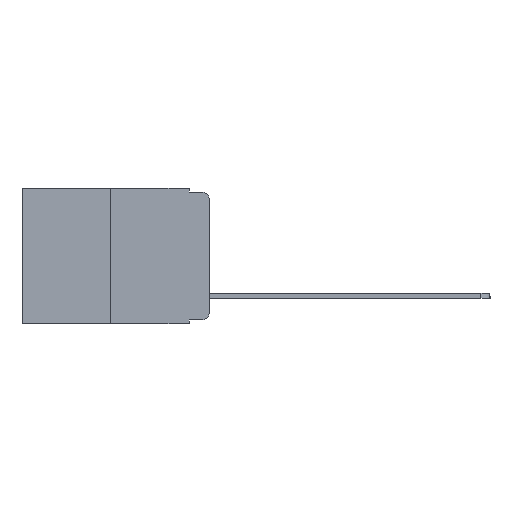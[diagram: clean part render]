
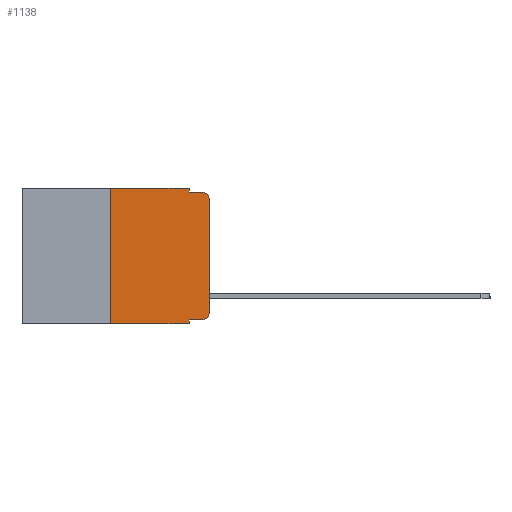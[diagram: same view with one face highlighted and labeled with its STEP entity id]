
A CAD part, left-side view. The second image highlights one B-rep face of the part: STEP entity #1138.
In plain terms, the highlighted planar face has unit normal (-1, 0, 0).
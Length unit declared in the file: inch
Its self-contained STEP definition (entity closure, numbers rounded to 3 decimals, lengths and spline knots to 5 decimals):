
#285 = VECTOR ( 'NONE', #13796, 39.37008 ) ;
#862 = ORIENTED_EDGE ( 'NONE', *, *, #1013, .T. ) ;
#1013 = EDGE_CURVE ( 'NONE', #11728, #10375, #12102, .T. ) ;
#1138 = ADVANCED_FACE ( 'NONE', ( #19565 ), #14277, .F. ) ;
#1579 = DIRECTION ( 'NONE',  ( -1., 0., 0. ) ) ;
#1779 = ORIENTED_EDGE ( 'NONE', *, *, #4696, .T. ) ;
#1938 = CARTESIAN_POINT ( 'NONE',  ( 0., 0.02, -0.333 ) ) ;
#2696 = EDGE_CURVE ( 'NONE', #3212, #5462, #18190, .T. ) ;
#2874 = CARTESIAN_POINT ( 'NONE',  ( 0., 0.051, -0.333 ) ) ;
#3212 = VERTEX_POINT ( 'NONE', #9689 ) ;
#3411 = DIRECTION ( 'NONE',  ( 0., 0., -1. ) ) ;
#3499 = DIRECTION ( 'NONE',  ( 0., 0., -1. ) ) ;
#3868 = DIRECTION ( 'NONE',  ( 0., -1., 0. ) ) ;
#3967 = EDGE_CURVE ( 'NONE', #11728, #5462, #16290, .T. ) ;
#4648 = EDGE_CURVE ( 'NONE', #17706, #18360, #19106, .T. ) ;
#4696 = EDGE_CURVE ( 'NONE', #9581, #6731, #10165, .T. ) ;
#4700 = DIRECTION ( 'NONE',  ( 0., -1., 0. ) ) ;
#5462 = VERTEX_POINT ( 'NONE', #13153 ) ;
#6020 = EDGE_CURVE ( 'NONE', #19674, #21864, #15008, .T. ) ;
#6176 = CIRCLE ( 'NONE', #14310, 0.02 ) ;
#6731 = VERTEX_POINT ( 'NONE', #9118 ) ;
#6762 = VECTOR ( 'NONE', #3499, 39.37008 ) ;
#6917 = CARTESIAN_POINT ( 'NONE',  ( 0., 0.051, 0. ) ) ;
#7297 = CARTESIAN_POINT ( 'NONE',  ( 0., 0.473, -0.343 ) ) ;
#7717 = ORIENTED_EDGE ( 'NONE', *, *, #3967, .F. ) ;
#8801 = CARTESIAN_POINT ( 'NONE',  ( 0., 0.051, 0. ) ) ;
#8881 = CARTESIAN_POINT ( 'NONE',  ( 0., 0.02, -0.03 ) ) ;
#9118 = CARTESIAN_POINT ( 'NONE',  ( 0., 0., -0.03 ) ) ;
#9581 = VERTEX_POINT ( 'NONE', #19631 ) ;
#9689 = CARTESIAN_POINT ( 'NONE',  ( 0., 0.25, -0.343 ) ) ;
#10165 = LINE ( 'NONE', #23197, #14858 ) ;
#10375 = VERTEX_POINT ( 'NONE', #1938 ) ;
#10949 = AXIS2_PLACEMENT_3D ( 'NONE', #19239, #17543, #11891 ) ;
#11382 = CARTESIAN_POINT ( 'NONE',  ( 0., 0.051, -0.01 ) ) ;
#11728 = VERTEX_POINT ( 'NONE', #20588 ) ;
#11891 = DIRECTION ( 'NONE',  ( 0., 0., -1. ) ) ;
#12102 = LINE ( 'NONE', #2874, #285 ) ;
#12781 = ORIENTED_EDGE ( 'NONE', *, *, #4648, .F. ) ;
#13079 = LINE ( 'NONE', #20424, #6762 ) ;
#13153 = CARTESIAN_POINT ( 'NONE',  ( 0., 0.051, -0.343 ) ) ;
#13265 = CIRCLE ( 'NONE', #10949, 0.02 ) ;
#13267 = VECTOR ( 'NONE', #4700, 39.37008 ) ;
#13796 = DIRECTION ( 'NONE',  ( 0., -1., 0. ) ) ;
#13826 = ORIENTED_EDGE ( 'NONE', *, *, #6020, .F. ) ;
#14277 = PLANE ( 'NONE',  #14624 ) ;
#14310 = AXIS2_PLACEMENT_3D ( 'NONE', #8881, #1579, #3411 ) ;
#14624 = AXIS2_PLACEMENT_3D ( 'NONE', #19685, #18133, #18010 ) ;
#14858 = VECTOR ( 'NONE', #22850, 39.37008 ) ;
#15008 = LINE ( 'NONE', #11382, #16898 ) ;
#15170 = VECTOR ( 'NONE', #18427, 39.37008 ) ;
#15509 = ORIENTED_EDGE ( 'NONE', *, *, #19591, .T. ) ;
#15558 = ORIENTED_EDGE ( 'NONE', *, *, #21041, .T. ) ;
#16172 = DIRECTION ( 'NONE',  ( 0., 0., -1. ) ) ;
#16290 = LINE ( 'NONE', #8801, #23010 ) ;
#16898 = VECTOR ( 'NONE', #3868, 39.37008 ) ;
#17286 = ORIENTED_EDGE ( 'NONE', *, *, #2696, .T. ) ;
#17518 = DIRECTION ( 'NONE',  ( 0., 0., 1. ) ) ;
#17543 = DIRECTION ( 'NONE',  ( -1., 0., 0. ) ) ;
#17706 = VERTEX_POINT ( 'NONE', #22329 ) ;
#18010 = DIRECTION ( 'NONE',  ( 0., 0., -1. ) ) ;
#18133 = DIRECTION ( 'NONE',  ( 1., 0., 0. ) ) ;
#18190 = LINE ( 'NONE', #7297, #15170 ) ;
#18292 = EDGE_LOOP ( 'NONE', ( #1779, #15509, #13826, #21531, #12781, #22753, #17286, #7717, #862, #15558 ) ) ;
#18360 = VERTEX_POINT ( 'NONE', #6917 ) ;
#18427 = DIRECTION ( 'NONE',  ( 0., -1., 0. ) ) ;
#19106 = LINE ( 'NONE', #22967, #13267 ) ;
#19239 = CARTESIAN_POINT ( 'NONE',  ( 0., 0.02, -0.313 ) ) ;
#19565 = FACE_OUTER_BOUND ( 'NONE', #18292, .T. ) ;
#19591 = EDGE_CURVE ( 'NONE', #6731, #21864, #6176, .T. ) ;
#19631 = CARTESIAN_POINT ( 'NONE',  ( 0., 0., -0.313 ) ) ;
#19674 = VERTEX_POINT ( 'NONE', #23363 ) ;
#19685 = CARTESIAN_POINT ( 'NONE',  ( 0., 0.473, 0. ) ) ;
#20424 = CARTESIAN_POINT ( 'NONE',  ( 0., 0.051, 0. ) ) ;
#20588 = CARTESIAN_POINT ( 'NONE',  ( 0., 0.051, -0.333 ) ) ;
#21041 = EDGE_CURVE ( 'NONE', #10375, #9581, #13265, .T. ) ;
#21129 = CARTESIAN_POINT ( 'NONE',  ( 0., 0.25, 0. ) ) ;
#21379 = CARTESIAN_POINT ( 'NONE',  ( 0., 0.02, -0.01 ) ) ;
#21531 = ORIENTED_EDGE ( 'NONE', *, *, #23327, .F. ) ;
#21864 = VERTEX_POINT ( 'NONE', #21379 ) ;
#22230 = VECTOR ( 'NONE', #17518, 39.37008 ) ;
#22329 = CARTESIAN_POINT ( 'NONE',  ( 0., 0.25, 0. ) ) ;
#22753 = ORIENTED_EDGE ( 'NONE', *, *, #23557, .F. ) ;
#22850 = DIRECTION ( 'NONE',  ( 0., 0., 1. ) ) ;
#22967 = CARTESIAN_POINT ( 'NONE',  ( 0., 0.473, 0. ) ) ;
#23010 = VECTOR ( 'NONE', #16172, 39.37008 ) ;
#23197 = CARTESIAN_POINT ( 'NONE',  ( 0., 0., 0. ) ) ;
#23304 = LINE ( 'NONE', #21129, #22230 ) ;
#23327 = EDGE_CURVE ( 'NONE', #18360, #19674, #13079, .T. ) ;
#23363 = CARTESIAN_POINT ( 'NONE',  ( 0., 0.051, -0.01 ) ) ;
#23557 = EDGE_CURVE ( 'NONE', #3212, #17706, #23304, .T. ) ;
